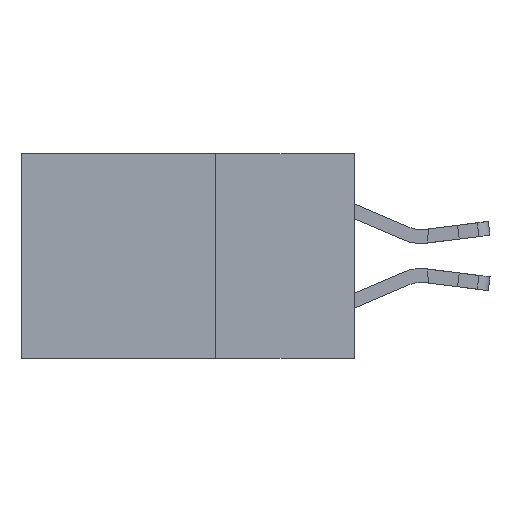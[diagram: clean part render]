
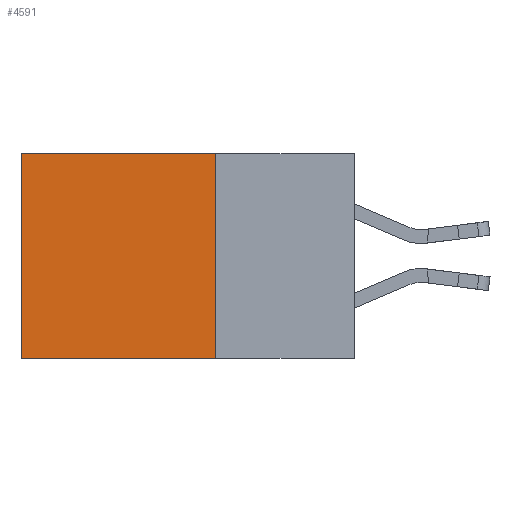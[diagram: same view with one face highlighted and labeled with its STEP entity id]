
A CAD part, left-side view. The second image highlights one B-rep face of the part: STEP entity #4591.
In plain terms, the highlighted planar face has unit normal (-1, 0, 0).
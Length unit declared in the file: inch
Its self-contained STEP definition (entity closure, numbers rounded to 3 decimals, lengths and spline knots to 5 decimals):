
#909 = VECTOR ( 'NONE', #5529, 39.37008 ) ;
#1012 = VERTEX_POINT ( 'NONE', #15853 ) ;
#1448 = EDGE_CURVE ( 'NONE', #4627, #1012, #6143, .T. ) ;
#2577 = DIRECTION ( 'NONE',  ( 0., 0., -1. ) ) ;
#2989 = DIRECTION ( 'NONE',  ( 0., 1., 0. ) ) ;
#3971 = AXIS2_PLACEMENT_3D ( 'NONE', #5957, #11157, #2577 ) ;
#4589 = ORIENTED_EDGE ( 'NONE', *, *, #17065, .F. ) ;
#4591 = ADVANCED_FACE ( 'NONE', ( #5225 ), #7505, .F. ) ;
#4627 = VERTEX_POINT ( 'NONE', #9449 ) ;
#5225 = FACE_OUTER_BOUND ( 'NONE', #10487, .T. ) ;
#5332 = ORIENTED_EDGE ( 'NONE', *, *, #6582, .T. ) ;
#5529 = DIRECTION ( 'NONE',  ( 0., 0., -1. ) ) ;
#5957 = CARTESIAN_POINT ( 'NONE',  ( 0.298, 0.25, 0. ) ) ;
#6143 = LINE ( 'NONE', #15271, #9588 ) ;
#6239 = VERTEX_POINT ( 'NONE', #9436 ) ;
#6582 = EDGE_CURVE ( 'NONE', #6239, #7580, #13620, .T. ) ;
#6850 = CARTESIAN_POINT ( 'NONE',  ( 0.298, 0.6, 0. ) ) ;
#7276 = LINE ( 'NONE', #14119, #10194 ) ;
#7380 = DIRECTION ( 'NONE',  ( 0., 1., 0. ) ) ;
#7505 = PLANE ( 'NONE',  #3971 ) ;
#7580 = VERTEX_POINT ( 'NONE', #17402 ) ;
#9436 = CARTESIAN_POINT ( 'NONE',  ( 0.298, 0.6, 0. ) ) ;
#9449 = CARTESIAN_POINT ( 'NONE',  ( 0.298, 0.25, 0. ) ) ;
#9588 = VECTOR ( 'NONE', #15567, 39.37008 ) ;
#10194 = VECTOR ( 'NONE', #7380, 39.37008 ) ;
#10487 = EDGE_LOOP ( 'NONE', ( #5332, #4589, #18225, #16598 ) ) ;
#11157 = DIRECTION ( 'NONE',  ( 1., 0., 0. ) ) ;
#13620 = LINE ( 'NONE', #6850, #909 ) ;
#14119 = CARTESIAN_POINT ( 'NONE',  ( 0.298, 0.25, -0.37 ) ) ;
#15271 = CARTESIAN_POINT ( 'NONE',  ( 0.298, 0.25, 0. ) ) ;
#15567 = DIRECTION ( 'NONE',  ( 0., 0., -1. ) ) ;
#15853 = CARTESIAN_POINT ( 'NONE',  ( 0.298, 0.25, -0.37 ) ) ;
#16007 = LINE ( 'NONE', #20380, #20250 ) ;
#16598 = ORIENTED_EDGE ( 'NONE', *, *, #16648, .T. ) ;
#16648 = EDGE_CURVE ( 'NONE', #4627, #6239, #16007, .T. ) ;
#17065 = EDGE_CURVE ( 'NONE', #1012, #7580, #7276, .T. ) ;
#17402 = CARTESIAN_POINT ( 'NONE',  ( 0.298, 0.6, -0.37 ) ) ;
#18225 = ORIENTED_EDGE ( 'NONE', *, *, #1448, .F. ) ;
#20250 = VECTOR ( 'NONE', #2989, 39.37008 ) ;
#20380 = CARTESIAN_POINT ( 'NONE',  ( 0.298, 0.25, 0. ) ) ;
